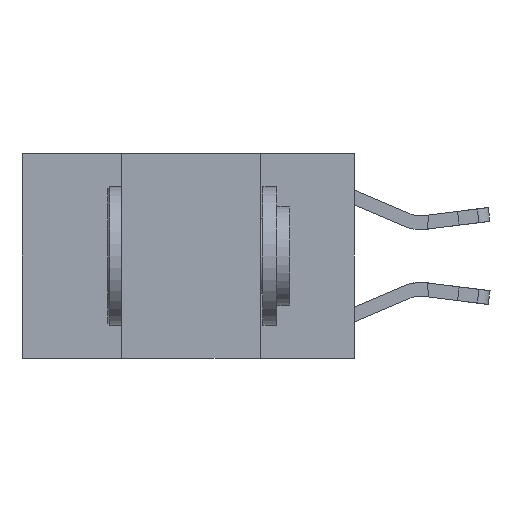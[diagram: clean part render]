
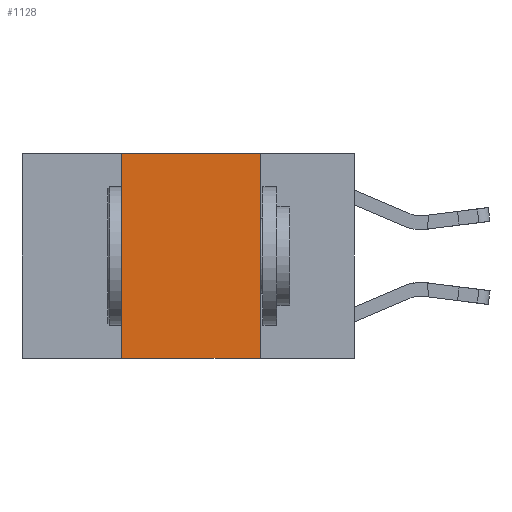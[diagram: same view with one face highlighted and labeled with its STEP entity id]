
A CAD part, left-side view. The second image highlights one B-rep face of the part: STEP entity #1128.
In plain terms, the highlighted planar face has unit normal (-1, 0, 0).
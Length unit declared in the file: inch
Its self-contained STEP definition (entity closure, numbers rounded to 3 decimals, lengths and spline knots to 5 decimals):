
#402 = LINE ( 'NONE', #11364, #24590 ) ;
#1128 = ADVANCED_FACE ( 'NONE', ( #24464 ), #3383, .F. ) ;
#2020 = EDGE_LOOP ( 'NONE', ( #21433, #11726, #3842, #16575 ) ) ;
#2138 = VECTOR ( 'NONE', #24066, 39.37008 ) ;
#2350 = EDGE_CURVE ( 'NONE', #25686, #24870, #17549, .T. ) ;
#3240 = EDGE_CURVE ( 'NONE', #10346, #25686, #402, .T. ) ;
#3383 = PLANE ( 'NONE',  #14483 ) ;
#3842 = ORIENTED_EDGE ( 'NONE', *, *, #19357, .F. ) ;
#5095 = CARTESIAN_POINT ( 'NONE',  ( 0., 0.42, 0. ) ) ;
#5596 = DIRECTION ( 'NONE',  ( 0., 0., -1. ) ) ;
#9890 = VERTEX_POINT ( 'NONE', #25124 ) ;
#10346 = VERTEX_POINT ( 'NONE', #25232 ) ;
#11364 = CARTESIAN_POINT ( 'NONE',  ( 0., 0.6, 0. ) ) ;
#11726 = ORIENTED_EDGE ( 'NONE', *, *, #3240, .F. ) ;
#14110 = VECTOR ( 'NONE', #23370, 39.37008 ) ;
#14483 = AXIS2_PLACEMENT_3D ( 'NONE', #20304, #24600, #5596 ) ;
#14910 = CARTESIAN_POINT ( 'NONE',  ( 0., 0.17, 0. ) ) ;
#15755 = EDGE_CURVE ( 'NONE', #9890, #24870, #17537, .T. ) ;
#16575 = ORIENTED_EDGE ( 'NONE', *, *, #15755, .T. ) ;
#17537 = LINE ( 'NONE', #21710, #14110 ) ;
#17549 = LINE ( 'NONE', #26011, #2138 ) ;
#19357 = EDGE_CURVE ( 'NONE', #9890, #10346, #26192, .T. ) ;
#20095 = DIRECTION ( 'NONE',  ( 0., -1., 0. ) ) ;
#20304 = CARTESIAN_POINT ( 'NONE',  ( 0., 0.6, 0. ) ) ;
#21433 = ORIENTED_EDGE ( 'NONE', *, *, #2350, .F. ) ;
#21710 = CARTESIAN_POINT ( 'NONE',  ( 0., 0.6, -0.37 ) ) ;
#23370 = DIRECTION ( 'NONE',  ( 0., -1., 0. ) ) ;
#23555 = DIRECTION ( 'NONE',  ( 0., 0., 1. ) ) ;
#24008 = CARTESIAN_POINT ( 'NONE',  ( 0., 0.17, -0.37 ) ) ;
#24066 = DIRECTION ( 'NONE',  ( 0., 0., -1. ) ) ;
#24464 = FACE_OUTER_BOUND ( 'NONE', #2020, .T. ) ;
#24590 = VECTOR ( 'NONE', #20095, 39.37008 ) ;
#24600 = DIRECTION ( 'NONE',  ( 1., 0., 0. ) ) ;
#24870 = VERTEX_POINT ( 'NONE', #24008 ) ;
#25124 = CARTESIAN_POINT ( 'NONE',  ( 0., 0.42, -0.37 ) ) ;
#25232 = CARTESIAN_POINT ( 'NONE',  ( 0., 0.42, 0. ) ) ;
#25686 = VERTEX_POINT ( 'NONE', #14910 ) ;
#25700 = VECTOR ( 'NONE', #23555, 39.37008 ) ;
#26011 = CARTESIAN_POINT ( 'NONE',  ( 0., 0.17, 0. ) ) ;
#26192 = LINE ( 'NONE', #5095, #25700 ) ;
